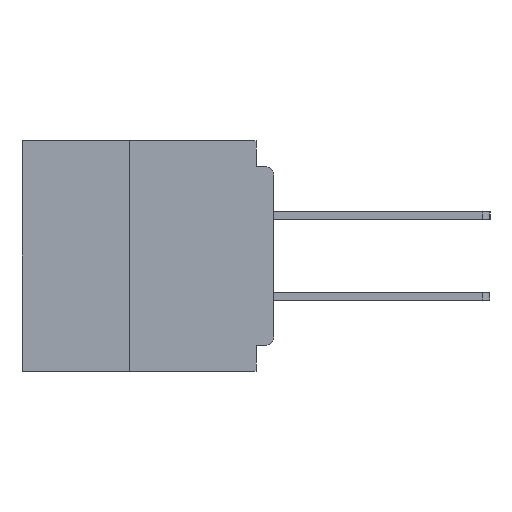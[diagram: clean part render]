
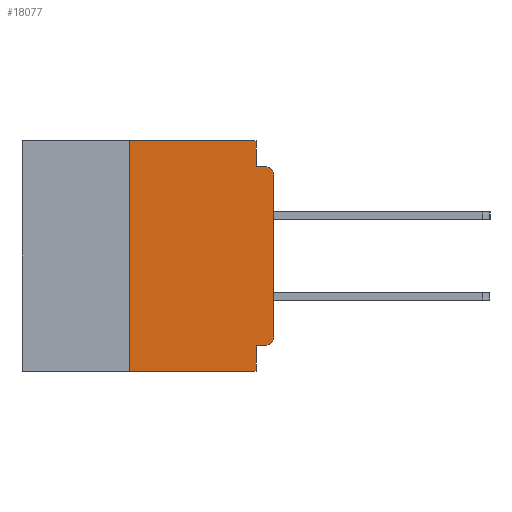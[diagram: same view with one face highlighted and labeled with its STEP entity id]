
A CAD part, left-side view. The second image highlights one B-rep face of the part: STEP entity #18077.
In plain terms, the highlighted planar face has unit normal (-1, 0, 0).
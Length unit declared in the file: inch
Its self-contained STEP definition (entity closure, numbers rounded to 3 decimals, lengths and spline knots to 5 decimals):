
#832 = CARTESIAN_POINT ( 'NONE',  ( 0., 0.031, 0. ) ) ;
#908 = ORIENTED_EDGE ( 'NONE', *, *, #7537, .T. ) ;
#1328 = CARTESIAN_POINT ( 'NONE',  ( 0., 0.031, -0.4 ) ) ;
#1352 = LINE ( 'NONE', #13909, #9499 ) ;
#1609 = VECTOR ( 'NONE', #6353, 39.37008 ) ;
#1750 = DIRECTION ( 'NONE',  ( 0., 1., 0. ) ) ;
#2850 = DIRECTION ( 'NONE',  ( 0., 0., -1. ) ) ;
#4600 = VERTEX_POINT ( 'NONE', #27114 ) ;
#5796 = DIRECTION ( 'NONE',  ( 1., 0., 0. ) ) ;
#5849 = LINE ( 'NONE', #16810, #29205 ) ;
#6234 = CARTESIAN_POINT ( 'NONE',  ( 0., 0.25, 0. ) ) ;
#6353 = DIRECTION ( 'NONE',  ( 0., -1., 0. ) ) ;
#7537 = EDGE_CURVE ( 'NONE', #9115, #10779, #32373, .T. ) ;
#8067 = CARTESIAN_POINT ( 'NONE',  ( 0., 0., -0.06 ) ) ;
#9070 = LINE ( 'NONE', #27392, #32388 ) ;
#9115 = VERTEX_POINT ( 'NONE', #37973 ) ;
#9499 = VECTOR ( 'NONE', #1750, 39.37008 ) ;
#9753 = LINE ( 'NONE', #18486, #1609 ) ;
#10042 = ORIENTED_EDGE ( 'NONE', *, *, #13117, .F. ) ;
#10203 = CARTESIAN_POINT ( 'NONE',  ( 0., 0.015, -0.06 ) ) ;
#10522 = ORIENTED_EDGE ( 'NONE', *, *, #23145, .F. ) ;
#10563 = ORIENTED_EDGE ( 'NONE', *, *, #30662, .F. ) ;
#10779 = VERTEX_POINT ( 'NONE', #8067 ) ;
#10938 = PLANE ( 'NONE',  #36653 ) ;
#10984 = ORIENTED_EDGE ( 'NONE', *, *, #26184, .T. ) ;
#11358 = EDGE_CURVE ( 'NONE', #24774, #4600, #21621, .T. ) ;
#11458 = DIRECTION ( 'NONE',  ( -1., 0., 0. ) ) ;
#12217 = DIRECTION ( 'NONE',  ( 0., 0., 1. ) ) ;
#12282 = EDGE_CURVE ( 'NONE', #27336, #25430, #26776, .T. ) ;
#12457 = ORIENTED_EDGE ( 'NONE', *, *, #12282, .F. ) ;
#12819 = CARTESIAN_POINT ( 'NONE',  ( 0., 0.437, 0. ) ) ;
#13117 = EDGE_CURVE ( 'NONE', #31844, #27336, #35674, .T. ) ;
#13286 = DIRECTION ( 'NONE',  ( 0., 0., -1. ) ) ;
#13641 = EDGE_CURVE ( 'NONE', #36864, #4600, #9753, .T. ) ;
#13909 = CARTESIAN_POINT ( 'NONE',  ( 0., 0., -0.355 ) ) ;
#14887 = ORIENTED_EDGE ( 'NONE', *, *, #17404, .F. ) ;
#16571 = DIRECTION ( 'NONE',  ( 0., 0., -1. ) ) ;
#16810 = CARTESIAN_POINT ( 'NONE',  ( 0., 0., -0.045 ) ) ;
#17404 = EDGE_CURVE ( 'NONE', #26689, #24774, #1352, .T. ) ;
#18077 = ADVANCED_FACE ( 'NONE', ( #24229 ), #10938, .F. ) ;
#18320 = AXIS2_PLACEMENT_3D ( 'NONE', #10203, #31498, #13286 ) ;
#18486 = CARTESIAN_POINT ( 'NONE',  ( 0., 0.437, -0.4 ) ) ;
#18729 = VECTOR ( 'NONE', #16571, 39.37008 ) ;
#18913 = DIRECTION ( 'NONE',  ( 0., -1., 0. ) ) ;
#20639 = ORIENTED_EDGE ( 'NONE', *, *, #24051, .T. ) ;
#21621 = LINE ( 'NONE', #1328, #18729 ) ;
#23145 = EDGE_CURVE ( 'NONE', #25430, #33939, #5849, .T. ) ;
#24051 = EDGE_CURVE ( 'NONE', #26689, #9115, #36206, .T. ) ;
#24202 = CARTESIAN_POINT ( 'NONE',  ( 0., 0.031, 0. ) ) ;
#24229 = FACE_OUTER_BOUND ( 'NONE', #31008, .T. ) ;
#24774 = VERTEX_POINT ( 'NONE', #30538 ) ;
#25430 = VERTEX_POINT ( 'NONE', #36687 ) ;
#26184 = EDGE_CURVE ( 'NONE', #10779, #33939, #37888, .T. ) ;
#26689 = VERTEX_POINT ( 'NONE', #36724 ) ;
#26776 = LINE ( 'NONE', #24202, #33838 ) ;
#26916 = CARTESIAN_POINT ( 'NONE',  ( 0., 0.015, -0.045 ) ) ;
#27114 = CARTESIAN_POINT ( 'NONE',  ( 0., 0.031, -0.4 ) ) ;
#27134 = DIRECTION ( 'NONE',  ( 0., 0., -1. ) ) ;
#27146 = CARTESIAN_POINT ( 'NONE',  ( 0., 0., 0. ) ) ;
#27336 = VERTEX_POINT ( 'NONE', #832 ) ;
#27392 = CARTESIAN_POINT ( 'NONE',  ( 0., 0.25, -0.4 ) ) ;
#27657 = VECTOR ( 'NONE', #18913, 39.37008 ) ;
#28664 = ORIENTED_EDGE ( 'NONE', *, *, #13641, .T. ) ;
#29205 = VECTOR ( 'NONE', #34958, 39.37008 ) ;
#29664 = CARTESIAN_POINT ( 'NONE',  ( 0., 0.015, -0.34 ) ) ;
#30180 = DIRECTION ( 'NONE',  ( 0., 0., 1. ) ) ;
#30538 = CARTESIAN_POINT ( 'NONE',  ( 0., 0.031, -0.355 ) ) ;
#30662 = EDGE_CURVE ( 'NONE', #36864, #31844, #9070, .T. ) ;
#31008 = EDGE_LOOP ( 'NONE', ( #908, #10984, #10522, #12457, #10042, #10563, #28664, #36229, #14887, #20639 ) ) ;
#31498 = DIRECTION ( 'NONE',  ( -1., 0., 0. ) ) ;
#31844 = VERTEX_POINT ( 'NONE', #6234 ) ;
#32373 = LINE ( 'NONE', #27146, #38487 ) ;
#32388 = VECTOR ( 'NONE', #12217, 39.37008 ) ;
#32715 = DIRECTION ( 'NONE',  ( 0., 0., -1. ) ) ;
#33838 = VECTOR ( 'NONE', #2850, 39.37008 ) ;
#33939 = VERTEX_POINT ( 'NONE', #26916 ) ;
#34512 = AXIS2_PLACEMENT_3D ( 'NONE', #29664, #11458, #32715 ) ;
#34958 = DIRECTION ( 'NONE',  ( 0., -1., 0. ) ) ;
#35087 = CARTESIAN_POINT ( 'NONE',  ( 0., 0.437, 0. ) ) ;
#35674 = LINE ( 'NONE', #12819, #27657 ) ;
#36206 = CIRCLE ( 'NONE', #34512, 0.015 ) ;
#36229 = ORIENTED_EDGE ( 'NONE', *, *, #11358, .F. ) ;
#36653 = AXIS2_PLACEMENT_3D ( 'NONE', #35087, #5796, #27134 ) ;
#36687 = CARTESIAN_POINT ( 'NONE',  ( 0., 0.031, -0.045 ) ) ;
#36724 = CARTESIAN_POINT ( 'NONE',  ( 0., 0.015, -0.355 ) ) ;
#36864 = VERTEX_POINT ( 'NONE', #38078 ) ;
#37888 = CIRCLE ( 'NONE', #18320, 0.015 ) ;
#37973 = CARTESIAN_POINT ( 'NONE',  ( 0., 0., -0.34 ) ) ;
#38078 = CARTESIAN_POINT ( 'NONE',  ( 0., 0.25, -0.4 ) ) ;
#38487 = VECTOR ( 'NONE', #30180, 39.37008 ) ;
